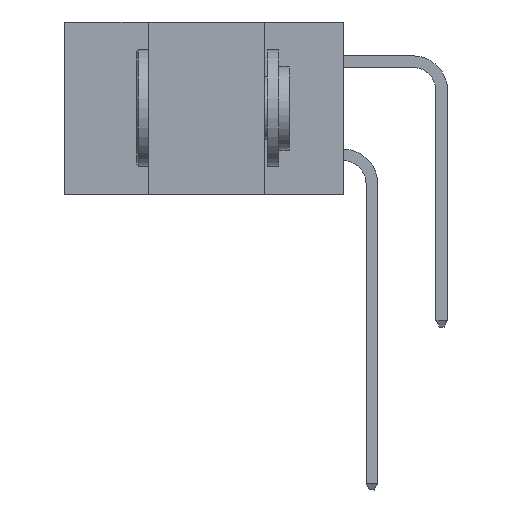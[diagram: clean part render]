
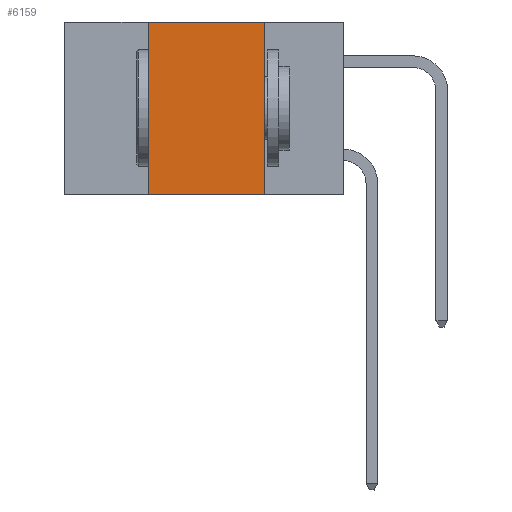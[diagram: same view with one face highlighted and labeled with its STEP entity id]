
A CAD part, left-side view. The second image highlights one B-rep face of the part: STEP entity #6159.
In plain terms, the highlighted planar face has unit normal (-1, 0, 0).
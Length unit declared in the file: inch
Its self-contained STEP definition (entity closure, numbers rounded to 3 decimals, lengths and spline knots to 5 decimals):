
#636 = VERTEX_POINT ( 'NONE', #4138 ) ;
#667 = LINE ( 'NONE', #1668, #7063 ) ;
#743 = VERTEX_POINT ( 'NONE', #9522 ) ;
#745 = EDGE_CURVE ( 'NONE', #4189, #11666, #3554, .T. ) ;
#989 = AXIS2_PLACEMENT_3D ( 'NONE', #7790, #9706, #1676 ) ;
#1287 = VECTOR ( 'NONE', #2876, 39.37008 ) ;
#1334 = ORIENTED_EDGE ( 'NONE', *, *, #7861, .F. ) ;
#1668 = CARTESIAN_POINT ( 'NONE',  ( 0., 0.42, -0.37 ) ) ;
#1676 = DIRECTION ( 'NONE',  ( 0., 0., -1. ) ) ;
#1910 = CARTESIAN_POINT ( 'NONE',  ( 0., 0.17, 0. ) ) ;
#2192 = ORIENTED_EDGE ( 'NONE', *, *, #9025, .T. ) ;
#2384 = DIRECTION ( 'NONE',  ( 0., -1., 0. ) ) ;
#2582 = ORIENTED_EDGE ( 'NONE', *, *, #745, .F. ) ;
#2876 = DIRECTION ( 'NONE',  ( 0., -1., 0. ) ) ;
#3554 = LINE ( 'NONE', #5476, #8790 ) ;
#3797 = CARTESIAN_POINT ( 'NONE',  ( 0., 0.6, 0. ) ) ;
#3807 = PLANE ( 'NONE',  #989 ) ;
#3944 = EDGE_CURVE ( 'NONE', #636, #743, #667, .T. ) ;
#4138 = CARTESIAN_POINT ( 'NONE',  ( 0., 0.42, -0.37 ) ) ;
#4189 = VERTEX_POINT ( 'NONE', #1910 ) ;
#4777 = CARTESIAN_POINT ( 'NONE',  ( 0., 0.17, -0.37 ) ) ;
#5476 = CARTESIAN_POINT ( 'NONE',  ( 0., 0.17, -0.37 ) ) ;
#6159 = ADVANCED_FACE ( 'NONE', ( #10462 ), #3807, .F. ) ;
#7063 = VECTOR ( 'NONE', #10387, 39.37008 ) ;
#7790 = CARTESIAN_POINT ( 'NONE',  ( 0., 0.6, 0. ) ) ;
#7861 = EDGE_CURVE ( 'NONE', #743, #4189, #11674, .T. ) ;
#8616 = ORIENTED_EDGE ( 'NONE', *, *, #3944, .F. ) ;
#8790 = VECTOR ( 'NONE', #10478, 39.37008 ) ;
#9025 = EDGE_CURVE ( 'NONE', #636, #11666, #11175, .T. ) ;
#9361 = VECTOR ( 'NONE', #2384, 39.37008 ) ;
#9522 = CARTESIAN_POINT ( 'NONE',  ( 0., 0.42, 0. ) ) ;
#9706 = DIRECTION ( 'NONE',  ( 1., 0., 0. ) ) ;
#10152 = CARTESIAN_POINT ( 'NONE',  ( 0., 0.6, -0.37 ) ) ;
#10387 = DIRECTION ( 'NONE',  ( 0., 0., 1. ) ) ;
#10462 = FACE_OUTER_BOUND ( 'NONE', #11932, .T. ) ;
#10478 = DIRECTION ( 'NONE',  ( 0., 0., -1. ) ) ;
#11175 = LINE ( 'NONE', #10152, #9361 ) ;
#11666 = VERTEX_POINT ( 'NONE', #4777 ) ;
#11674 = LINE ( 'NONE', #3797, #1287 ) ;
#11932 = EDGE_LOOP ( 'NONE', ( #2582, #1334, #8616, #2192 ) ) ;
